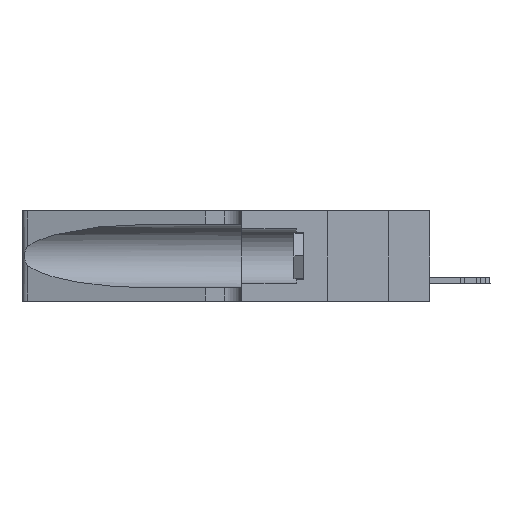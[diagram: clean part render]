
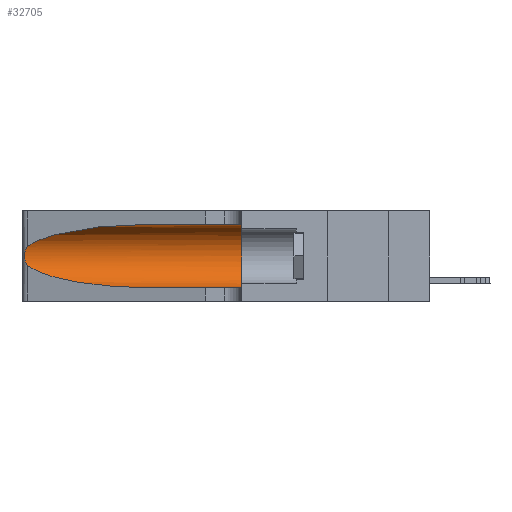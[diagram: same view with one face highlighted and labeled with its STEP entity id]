
A CAD part, left-side view. The second image highlights one B-rep face of the part: STEP entity #32705.
In plain terms, the highlighted cylindrical face has radius 3.308 mm (diameter 6.617 mm), a partial arc.
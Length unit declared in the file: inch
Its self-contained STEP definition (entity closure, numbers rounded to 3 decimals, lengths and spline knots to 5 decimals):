
#19 = EDGE_CURVE ( 'NONE', #29516, #23312, #13370, .T. ) ;
#667 = VECTOR ( 'NONE', #3269, 39.37008 ) ;
#1368 = CARTESIAN_POINT ( 'NONE',  ( 0.1305, 1.61858, 0.05475 ) ) ;
#2368 = AXIS2_PLACEMENT_3D ( 'NONE', #12996, #35995, #9260 ) ;
#3014 = VERTEX_POINT ( 'NONE', #27370 ) ;
#3269 = DIRECTION ( 'NONE',  ( 0., -1., 0. ) ) ;
#3862 = CARTESIAN_POINT ( 'NONE',  ( 0.26017, 1.23833, 0.17102 ) ) ;
#4146 = CARTESIAN_POINT ( 'NONE',  ( 0.25854, 1.2359, 0.20912 ) ) ;
#4291 = CARTESIAN_POINT ( 'NONE',  ( 0.25789, 1.23486, 0.15765 ) ) ;
#5496 = ORIENTED_EDGE ( 'NONE', *, *, #30688, .F. ) ;
#5628 = CARTESIAN_POINT ( 'NONE',  ( 0.18966, 0.96281, 0.31525 ) ) ;
#5836 =( BOUNDED_CURVE ( )  B_SPLINE_CURVE ( 3, ( #15312, #5628, #38633, #32021 ),
 .UNSPECIFIED., .F., .T. ) 
 B_SPLINE_CURVE_WITH_KNOTS ( ( 4, 4 ),
 ( 1.5708, 2.84003 ),
 .UNSPECIFIED. ) 
 CURVE ( )  GEOMETRIC_REPRESENTATION_ITEM ( )  RATIONAL_B_SPLINE_CURVE ( ( 1., 0.87, 0.87, 1. ) ) 
 REPRESENTATION_ITEM ( '' )  );
#7006 = CARTESIAN_POINT ( 'NONE',  ( 0.25487, 1.22718, 0.14631 ) ) ;
#7221 = EDGE_CURVE ( 'NONE', #20251, #29516, #5836, .T. ) ;
#7443 = CARTESIAN_POINT ( 'NONE',  ( 0.25555, 1.22993, 0.14849 ) ) ;
#7512 = CYLINDRICAL_SURFACE ( 'NONE', #14159, 0.13025 ) ;
#7585 = CARTESIAN_POINT ( 'NONE',  ( 0.25487, 1.22718, 0.14631 ) ) ;
#7756 = LINE ( 'NONE', #1368, #12390 ) ;
#8129 = CIRCLE ( 'NONE', #2368, 0.13025 ) ;
#9090 = EDGE_CURVE ( 'NONE', #20251, #36486, #32603, .T. ) ;
#9260 = DIRECTION ( 'NONE',  ( 0., 0., 1. ) ) ;
#10839 = CARTESIAN_POINT ( 'NONE',  ( 0.25787, 1.23484, 0.2124 ) ) ;
#11244 = DIRECTION ( 'NONE',  ( 0., 0., -1. ) ) ;
#12390 = VECTOR ( 'NONE', #25073, 39.37008 ) ;
#12996 = CARTESIAN_POINT ( 'NONE',  ( 0.1305, 0.35, 0.185 ) ) ;
#13032 = ORIENTED_EDGE ( 'NONE', *, *, #41225, .T. ) ;
#13370 = B_SPLINE_CURVE_WITH_KNOTS ( 'NONE', 3,
 ( #17132, #14022, #27252, #10839, #4146, #40014, #23918, #33438, #3862, #13731, #4291, #33882, #7443, #7585 ),
 .UNSPECIFIED., .F., .F.,
 ( 4, 2, 2, 2, 2, 2, 4 ),
 ( 0., 0.00027, 0.00053, 0.00107, 0.0016, 0.00187, 0.00214 ),
 .UNSPECIFIED. ) ;
#13731 = CARTESIAN_POINT ( 'NONE',  ( 0.25856, 1.23593, 0.16098 ) ) ;
#14022 = CARTESIAN_POINT ( 'NONE',  ( 0.25555, 1.22994, 0.2215 ) ) ;
#14158 = EDGE_LOOP ( 'NONE', ( #35888, #28463, #37174, #13032, #5496, #25734 ) ) ;
#14159 = AXIS2_PLACEMENT_3D ( 'NONE', #31103, #24758, #11244 ) ;
#14952 = CARTESIAN_POINT ( 'NONE',  ( 0.2373, 1.15595, 0.08982 ) ) ;
#15032 = CARTESIAN_POINT ( 'NONE',  ( 0.1305, 0.35, 0.31525 ) ) ;
#15312 = CARTESIAN_POINT ( 'NONE',  ( 0.1305, 0.72297, 0.31525 ) ) ;
#17132 = CARTESIAN_POINT ( 'NONE',  ( 0.25487, 1.22718, 0.22369 ) ) ;
#20251 = VERTEX_POINT ( 'NONE', #35991 ) ;
#21513 = CARTESIAN_POINT ( 'NONE',  ( 0.1305, 0.72297, 0.05475 ) ) ;
#23312 = VERTEX_POINT ( 'NONE', #7006 ) ;
#23918 = CARTESIAN_POINT ( 'NONE',  ( 0.26075, 1.23896, 0.19203 ) ) ;
#24758 = DIRECTION ( 'NONE',  ( 0., -1., 0. ) ) ;
#25073 = DIRECTION ( 'NONE',  ( 0., -1., 0. ) ) ;
#25734 = ORIENTED_EDGE ( 'NONE', *, *, #9090, .F. ) ;
#27252 = CARTESIAN_POINT ( 'NONE',  ( 0.25639, 1.23184, 0.21858 ) ) ;
#27370 = CARTESIAN_POINT ( 'NONE',  ( 0.1305, 0.72297, 0.05475 ) ) ;
#28463 = ORIENTED_EDGE ( 'NONE', *, *, #19, .T. ) ;
#29362 = EDGE_CURVE ( 'NONE', #23312, #3014, #30483, .T. ) ;
#29516 = VERTEX_POINT ( 'NONE', #42396 ) ;
#30483 =( BOUNDED_CURVE ( )  B_SPLINE_CURVE ( 3, ( #34516, #14952, #37988, #21513 ),
 .UNSPECIFIED., .F., .T. ) 
 B_SPLINE_CURVE_WITH_KNOTS ( ( 4, 4 ),
 ( 3.44316, 4.71239 ),
 .UNSPECIFIED. ) 
 CURVE ( )  GEOMETRIC_REPRESENTATION_ITEM ( )  RATIONAL_B_SPLINE_CURVE ( ( 1., 0.87, 0.87, 1. ) ) 
 REPRESENTATION_ITEM ( '' )  );
#30688 = EDGE_CURVE ( 'NONE', #36486, #35350, #8129, .T. ) ;
#31103 = CARTESIAN_POINT ( 'NONE',  ( 0.1305, 1.61858, 0.185 ) ) ;
#31856 = CARTESIAN_POINT ( 'NONE',  ( 0.1305, 0.35, 0.05475 ) ) ;
#32021 = CARTESIAN_POINT ( 'NONE',  ( 0.25487, 1.22718, 0.22369 ) ) ;
#32603 = LINE ( 'NONE', #36535, #667 ) ;
#32705 = ADVANCED_FACE ( 'NONE', ( #40385 ), #7512, .F. ) ;
#33438 = CARTESIAN_POINT ( 'NONE',  ( 0.26075, 1.23896, 0.178 ) ) ;
#33882 = CARTESIAN_POINT ( 'NONE',  ( 0.25639, 1.23186, 0.15144 ) ) ;
#34516 = CARTESIAN_POINT ( 'NONE',  ( 0.25487, 1.22718, 0.14631 ) ) ;
#35350 = VERTEX_POINT ( 'NONE', #31856 ) ;
#35888 = ORIENTED_EDGE ( 'NONE', *, *, #7221, .T. ) ;
#35991 = CARTESIAN_POINT ( 'NONE',  ( 0.1305, 0.72297, 0.31525 ) ) ;
#35995 = DIRECTION ( 'NONE',  ( 0., 1., 0. ) ) ;
#36486 = VERTEX_POINT ( 'NONE', #15032 ) ;
#36535 = CARTESIAN_POINT ( 'NONE',  ( 0.1305, 1.61858, 0.31525 ) ) ;
#37174 = ORIENTED_EDGE ( 'NONE', *, *, #29362, .T. ) ;
#37988 = CARTESIAN_POINT ( 'NONE',  ( 0.18966, 0.96281, 0.05475 ) ) ;
#38633 = CARTESIAN_POINT ( 'NONE',  ( 0.2373, 1.15595, 0.28018 ) ) ;
#40014 = CARTESIAN_POINT ( 'NONE',  ( 0.26018, 1.23835, 0.19895 ) ) ;
#40385 = FACE_OUTER_BOUND ( 'NONE', #14158, .T. ) ;
#41225 = EDGE_CURVE ( 'NONE', #3014, #35350, #7756, .T. ) ;
#42396 = CARTESIAN_POINT ( 'NONE',  ( 0.25487, 1.22718, 0.22369 ) ) ;
